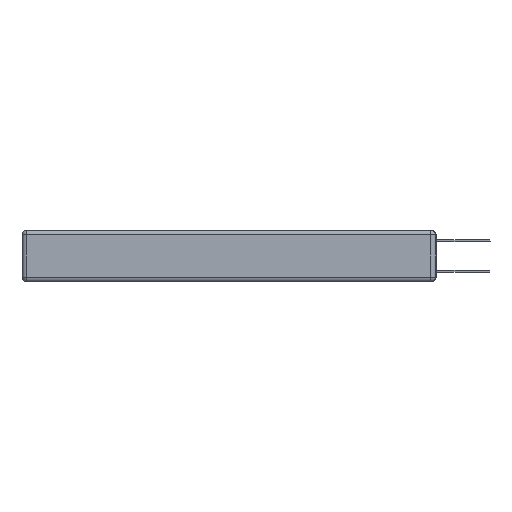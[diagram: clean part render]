
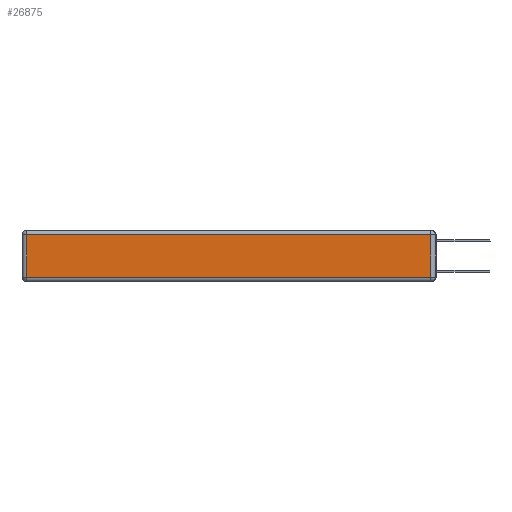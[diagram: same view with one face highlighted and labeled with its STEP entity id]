
A CAD part, left-side view. The second image highlights one B-rep face of the part: STEP entity #26875.
In plain terms, the highlighted planar face has unit normal (-1, 0, 0).
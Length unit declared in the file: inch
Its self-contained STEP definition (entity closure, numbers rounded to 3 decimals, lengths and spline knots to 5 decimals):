
#489 = EDGE_CURVE ( 'NONE', #22670, #22806, #21228, .T. ) ;
#3534 = CARTESIAN_POINT ( 'NONE',  ( 0., 0.03, -0.03 ) ) ;
#3768 = ORIENTED_EDGE ( 'NONE', *, *, #9886, .T. ) ;
#4873 = AXIS2_PLACEMENT_3D ( 'NONE', #26434, #13710, #22092 ) ;
#4994 = PLANE ( 'NONE',  #4873 ) ;
#5097 = LINE ( 'NONE', #24643, #19511 ) ;
#6377 = LINE ( 'NONE', #18721, #12751 ) ;
#6753 = CARTESIAN_POINT ( 'NONE',  ( 0., 0., -0.313 ) ) ;
#7312 = CARTESIAN_POINT ( 'NONE',  ( 0., 0.03, -0.313 ) ) ;
#8303 = LINE ( 'NONE', #21771, #23445 ) ;
#9614 = CARTESIAN_POINT ( 'NONE',  ( 0., 2.72, -0.313 ) ) ;
#9886 = EDGE_CURVE ( 'NONE', #15623, #11643, #5097, .T. ) ;
#10805 = DIRECTION ( 'NONE',  ( 0., 0., 1. ) ) ;
#11112 = VECTOR ( 'NONE', #13394, 39.37008 ) ;
#11643 = VERTEX_POINT ( 'NONE', #20457 ) ;
#11723 = DIRECTION ( 'NONE',  ( 0., 1., 0. ) ) ;
#11998 = EDGE_LOOP ( 'NONE', ( #16394, #18102, #3768, #17234 ) ) ;
#12751 = VECTOR ( 'NONE', #10805, 39.37008 ) ;
#13394 = DIRECTION ( 'NONE',  ( 0., -1., 0. ) ) ;
#13710 = DIRECTION ( 'NONE',  ( -1., 0., 0. ) ) ;
#15262 = EDGE_CURVE ( 'NONE', #11643, #22670, #8303, .T. ) ;
#15623 = VERTEX_POINT ( 'NONE', #3534 ) ;
#16321 = EDGE_CURVE ( 'NONE', #22806, #15623, #6377, .T. ) ;
#16394 = ORIENTED_EDGE ( 'NONE', *, *, #489, .T. ) ;
#17234 = ORIENTED_EDGE ( 'NONE', *, *, #15262, .T. ) ;
#18102 = ORIENTED_EDGE ( 'NONE', *, *, #16321, .T. ) ;
#18721 = CARTESIAN_POINT ( 'NONE',  ( 0., 0.03, -0.343 ) ) ;
#19511 = VECTOR ( 'NONE', #11723, 39.37008 ) ;
#19586 = FACE_OUTER_BOUND ( 'NONE', #11998, .T. ) ;
#19874 = DIRECTION ( 'NONE',  ( 0., 0., -1. ) ) ;
#20457 = CARTESIAN_POINT ( 'NONE',  ( 0., 2.72, -0.03 ) ) ;
#21228 = LINE ( 'NONE', #6753, #11112 ) ;
#21771 = CARTESIAN_POINT ( 'NONE',  ( 0., 2.72, -0.343 ) ) ;
#22092 = DIRECTION ( 'NONE',  ( 0., 0., 1. ) ) ;
#22670 = VERTEX_POINT ( 'NONE', #9614 ) ;
#22806 = VERTEX_POINT ( 'NONE', #7312 ) ;
#23445 = VECTOR ( 'NONE', #19874, 39.37008 ) ;
#24643 = CARTESIAN_POINT ( 'NONE',  ( 0., 2.75, -0.03 ) ) ;
#26434 = CARTESIAN_POINT ( 'NONE',  ( 0., 0., -0.343 ) ) ;
#26875 = ADVANCED_FACE ( 'NONE', ( #19586 ), #4994, .T. ) ;
